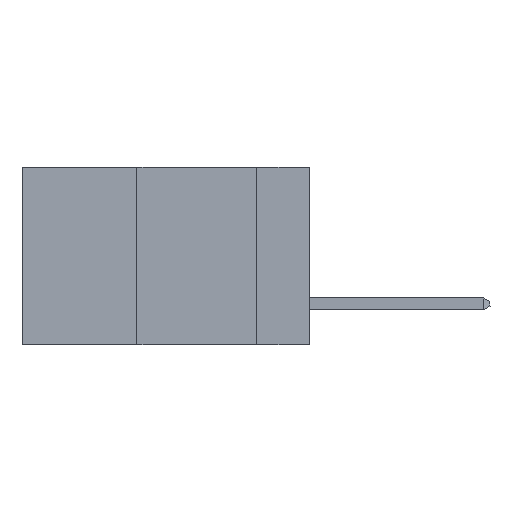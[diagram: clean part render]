
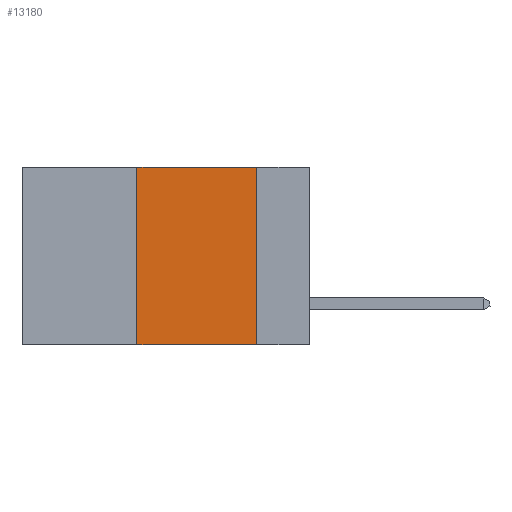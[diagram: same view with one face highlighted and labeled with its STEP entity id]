
A CAD part, left-side view. The second image highlights one B-rep face of the part: STEP entity #13180.
In plain terms, the highlighted planar face has unit normal (-1, 0, 0).
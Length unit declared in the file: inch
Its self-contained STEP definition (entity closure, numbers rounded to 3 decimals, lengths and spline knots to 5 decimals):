
#565 = VECTOR ( 'NONE', #3118, 39.37008 ) ;
#726 = DIRECTION ( 'NONE',  ( 0., 0., -1. ) ) ;
#1313 = ORIENTED_EDGE ( 'NONE', *, *, #4270, .F. ) ;
#1336 = EDGE_LOOP ( 'NONE', ( #1313, #1467, #1559, #1675 ) ) ;
#1397 = CARTESIAN_POINT ( 'NONE',  ( 0., 0.36, 0. ) ) ;
#1433 = VECTOR ( 'NONE', #13687, 39.37008 ) ;
#1467 = ORIENTED_EDGE ( 'NONE', *, *, #13151, .F. ) ;
#1522 = DIRECTION ( 'NONE',  ( 0., 0., 1. ) ) ;
#1559 = ORIENTED_EDGE ( 'NONE', *, *, #3474, .F. ) ;
#1619 = VERTEX_POINT ( 'NONE', #11861 ) ;
#1675 = ORIENTED_EDGE ( 'NONE', *, *, #1901, .T. ) ;
#1830 = CARTESIAN_POINT ( 'NONE',  ( 0., 0.36, -0.37 ) ) ;
#1877 = CARTESIAN_POINT ( 'NONE',  ( 0., 0.36, 0. ) ) ;
#1901 = EDGE_CURVE ( 'NONE', #7917, #4533, #4577, .T. ) ;
#2968 = VERTEX_POINT ( 'NONE', #1397 ) ;
#3118 = DIRECTION ( 'NONE',  ( 0., -1., 0. ) ) ;
#3474 = EDGE_CURVE ( 'NONE', #7917, #2968, #4365, .T. ) ;
#4270 = EDGE_CURVE ( 'NONE', #1619, #4533, #7718, .T. ) ;
#4303 = CARTESIAN_POINT ( 'NONE',  ( 0., 0.11, 0. ) ) ;
#4307 = CARTESIAN_POINT ( 'NONE',  ( 0., 0.6, 0. ) ) ;
#4365 = LINE ( 'NONE', #1877, #7049 ) ;
#4533 = VERTEX_POINT ( 'NONE', #9203 ) ;
#4577 = LINE ( 'NONE', #13728, #1433 ) ;
#4679 = VECTOR ( 'NONE', #726, 39.37008 ) ;
#6122 = FACE_OUTER_BOUND ( 'NONE', #1336, .T. ) ;
#6664 = CARTESIAN_POINT ( 'NONE',  ( 0., 0.6, 0. ) ) ;
#7049 = VECTOR ( 'NONE', #1522, 39.37008 ) ;
#7718 = LINE ( 'NONE', #4303, #4679 ) ;
#7766 = DIRECTION ( 'NONE',  ( 0., 0., -1. ) ) ;
#7917 = VERTEX_POINT ( 'NONE', #1830 ) ;
#9203 = CARTESIAN_POINT ( 'NONE',  ( 0., 0.11, -0.37 ) ) ;
#9707 = LINE ( 'NONE', #4307, #565 ) ;
#9876 = PLANE ( 'NONE',  #11290 ) ;
#11290 = AXIS2_PLACEMENT_3D ( 'NONE', #6664, #14030, #7766 ) ;
#11861 = CARTESIAN_POINT ( 'NONE',  ( 0., 0.11, 0. ) ) ;
#13151 = EDGE_CURVE ( 'NONE', #2968, #1619, #9707, .T. ) ;
#13180 = ADVANCED_FACE ( 'NONE', ( #6122 ), #9876, .F. ) ;
#13687 = DIRECTION ( 'NONE',  ( 0., -1., 0. ) ) ;
#13728 = CARTESIAN_POINT ( 'NONE',  ( 0., 0.6, -0.37 ) ) ;
#14030 = DIRECTION ( 'NONE',  ( 1., 0., 0. ) ) ;
